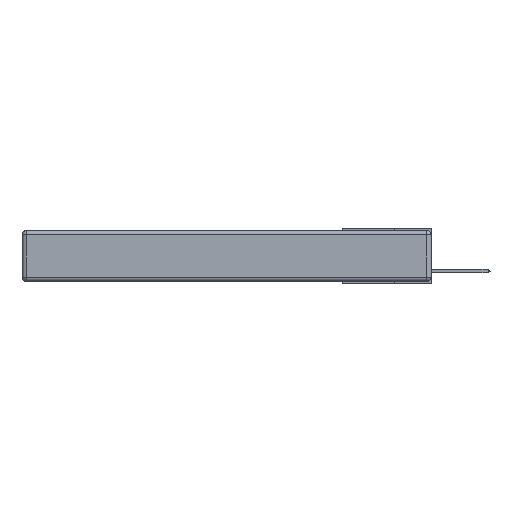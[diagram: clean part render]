
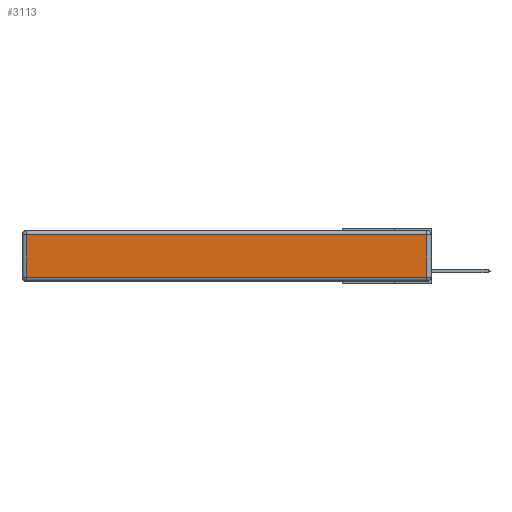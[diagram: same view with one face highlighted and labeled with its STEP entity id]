
A CAD part, left-side view. The second image highlights one B-rep face of the part: STEP entity #3113.
In plain terms, the highlighted planar face has unit normal (-1, 0, 0).
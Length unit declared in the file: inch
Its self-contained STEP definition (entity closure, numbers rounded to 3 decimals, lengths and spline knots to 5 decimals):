
#5 = EDGE_CURVE ( 'NONE', #7428, #13642, #1166, .T. ) ;
#290 = DIRECTION ( 'NONE',  ( -1., 0., 0. ) ) ;
#1166 = LINE ( 'NONE', #4218, #6862 ) ;
#1374 = DIRECTION ( 'NONE',  ( 0., 0., 1. ) ) ;
#1565 = ORIENTED_EDGE ( 'NONE', *, *, #5, .T. ) ;
#1673 = DIRECTION ( 'NONE',  ( 0., 0., 1. ) ) ;
#2245 = FACE_OUTER_BOUND ( 'NONE', #17896, .T. ) ;
#2306 = EDGE_CURVE ( 'NONE', #13642, #13124, #16919, .T. ) ;
#2906 = CARTESIAN_POINT ( 'NONE',  ( 0., 2.72, -0.313 ) ) ;
#2925 = DIRECTION ( 'NONE',  ( 0., 0., -1. ) ) ;
#3113 = ADVANCED_FACE ( 'NONE', ( #2245 ), #10132, .T. ) ;
#3370 = VECTOR ( 'NONE', #15271, 39.37008 ) ;
#4132 = ORIENTED_EDGE ( 'NONE', *, *, #2306, .T. ) ;
#4218 = CARTESIAN_POINT ( 'NONE',  ( 0., 2.72, -0.343 ) ) ;
#5222 = AXIS2_PLACEMENT_3D ( 'NONE', #7196, #290, #1673 ) ;
#5360 = ORIENTED_EDGE ( 'NONE', *, *, #10541, .T. ) ;
#5801 = CARTESIAN_POINT ( 'NONE',  ( 0., 0.03, -0.313 ) ) ;
#6862 = VECTOR ( 'NONE', #2925, 39.37008 ) ;
#7196 = CARTESIAN_POINT ( 'NONE',  ( 0., 0., -0.343 ) ) ;
#7371 = VECTOR ( 'NONE', #1374, 39.37008 ) ;
#7428 = VERTEX_POINT ( 'NONE', #17456 ) ;
#8002 = EDGE_CURVE ( 'NONE', #12350, #7428, #11626, .T. ) ;
#8686 = DIRECTION ( 'NONE',  ( 0., 1., 0. ) ) ;
#10132 = PLANE ( 'NONE',  #5222 ) ;
#10541 = EDGE_CURVE ( 'NONE', #13124, #12350, #12156, .T. ) ;
#10733 = CARTESIAN_POINT ( 'NONE',  ( 0., 0.03, -0.03 ) ) ;
#11360 = CARTESIAN_POINT ( 'NONE',  ( 0., 0.03, -0.343 ) ) ;
#11626 = LINE ( 'NONE', #13050, #13576 ) ;
#12156 = LINE ( 'NONE', #11360, #7371 ) ;
#12350 = VERTEX_POINT ( 'NONE', #10733 ) ;
#13023 = ORIENTED_EDGE ( 'NONE', *, *, #8002, .T. ) ;
#13050 = CARTESIAN_POINT ( 'NONE',  ( 0., 2.75, -0.03 ) ) ;
#13124 = VERTEX_POINT ( 'NONE', #5801 ) ;
#13576 = VECTOR ( 'NONE', #8686, 39.37008 ) ;
#13642 = VERTEX_POINT ( 'NONE', #2906 ) ;
#15271 = DIRECTION ( 'NONE',  ( 0., -1., 0. ) ) ;
#16553 = CARTESIAN_POINT ( 'NONE',  ( 0., 0., -0.313 ) ) ;
#16919 = LINE ( 'NONE', #16553, #3370 ) ;
#17456 = CARTESIAN_POINT ( 'NONE',  ( 0., 2.72, -0.03 ) ) ;
#17896 = EDGE_LOOP ( 'NONE', ( #4132, #5360, #13023, #1565 ) ) ;
